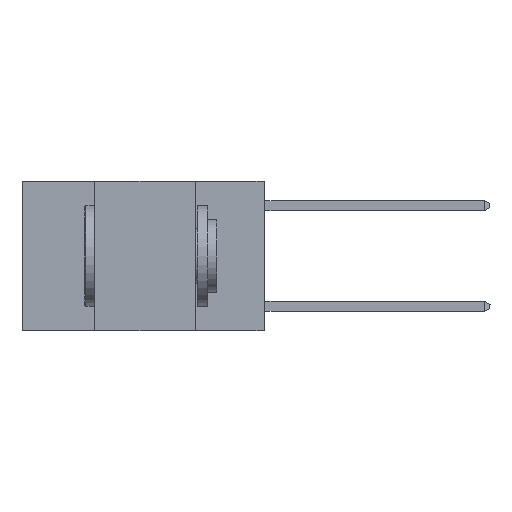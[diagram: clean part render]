
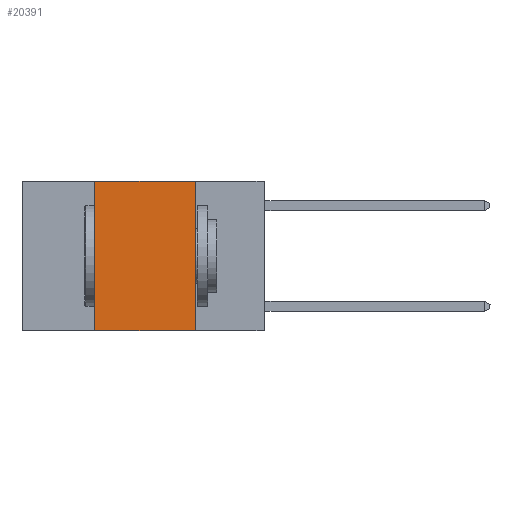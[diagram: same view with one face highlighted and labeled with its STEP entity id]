
A CAD part, left-side view. The second image highlights one B-rep face of the part: STEP entity #20391.
In plain terms, the highlighted planar face has unit normal (-1, 0, 0).
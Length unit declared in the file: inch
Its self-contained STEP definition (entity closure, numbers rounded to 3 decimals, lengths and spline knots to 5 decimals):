
#556 = VERTEX_POINT ( 'NONE', #6294 ) ;
#733 = EDGE_CURVE ( 'NONE', #8813, #11881, #20738, .T. ) ;
#1072 = DIRECTION ( 'NONE',  ( 0., 0., 1. ) ) ;
#2195 = VECTOR ( 'NONE', #21098, 39.37008 ) ;
#3408 = LINE ( 'NONE', #17312, #22493 ) ;
#3535 = PLANE ( 'NONE',  #11739 ) ;
#5696 = VERTEX_POINT ( 'NONE', #17341 ) ;
#6294 = CARTESIAN_POINT ( 'NONE',  ( 0., 0.42, -0.37 ) ) ;
#6771 = DIRECTION ( 'NONE',  ( 0., 0., -1. ) ) ;
#7049 = DIRECTION ( 'NONE',  ( 0., 0., -1. ) ) ;
#8813 = VERTEX_POINT ( 'NONE', #11932 ) ;
#9603 = VECTOR ( 'NONE', #1072, 39.37008 ) ;
#9995 = EDGE_CURVE ( 'NONE', #11881, #5696, #3408, .T. ) ;
#11739 = AXIS2_PLACEMENT_3D ( 'NONE', #15770, #17507, #7049 ) ;
#11747 = EDGE_CURVE ( 'NONE', #556, #8813, #18879, .T. ) ;
#11818 = CARTESIAN_POINT ( 'NONE',  ( 0., 0.17, 0. ) ) ;
#11881 = VERTEX_POINT ( 'NONE', #11818 ) ;
#11932 = CARTESIAN_POINT ( 'NONE',  ( 0., 0.42, 0. ) ) ;
#12116 = ORIENTED_EDGE ( 'NONE', *, *, #9995, .F. ) ;
#12621 = EDGE_LOOP ( 'NONE', ( #12116, #17296, #21912, #22439 ) ) ;
#13199 = VECTOR ( 'NONE', #15479, 39.37008 ) ;
#14080 = EDGE_CURVE ( 'NONE', #556, #5696, #17855, .T. ) ;
#15479 = DIRECTION ( 'NONE',  ( 0., -1., 0. ) ) ;
#15770 = CARTESIAN_POINT ( 'NONE',  ( 0., 0.6, 0. ) ) ;
#17296 = ORIENTED_EDGE ( 'NONE', *, *, #733, .F. ) ;
#17312 = CARTESIAN_POINT ( 'NONE',  ( 0., 0.17, 0. ) ) ;
#17341 = CARTESIAN_POINT ( 'NONE',  ( 0., 0.17, -0.37 ) ) ;
#17507 = DIRECTION ( 'NONE',  ( 1., 0., 0. ) ) ;
#17855 = LINE ( 'NONE', #22373, #13199 ) ;
#18104 = FACE_OUTER_BOUND ( 'NONE', #12621, .T. ) ;
#18879 = LINE ( 'NONE', #21557, #9603 ) ;
#20391 = ADVANCED_FACE ( 'NONE', ( #18104 ), #3535, .F. ) ;
#20738 = LINE ( 'NONE', #21172, #2195 ) ;
#21098 = DIRECTION ( 'NONE',  ( 0., -1., 0. ) ) ;
#21172 = CARTESIAN_POINT ( 'NONE',  ( 0., 0.6, 0. ) ) ;
#21557 = CARTESIAN_POINT ( 'NONE',  ( 0., 0.42, 0. ) ) ;
#21912 = ORIENTED_EDGE ( 'NONE', *, *, #11747, .F. ) ;
#22373 = CARTESIAN_POINT ( 'NONE',  ( 0., 0.6, -0.37 ) ) ;
#22439 = ORIENTED_EDGE ( 'NONE', *, *, #14080, .T. ) ;
#22493 = VECTOR ( 'NONE', #6771, 39.37008 ) ;
